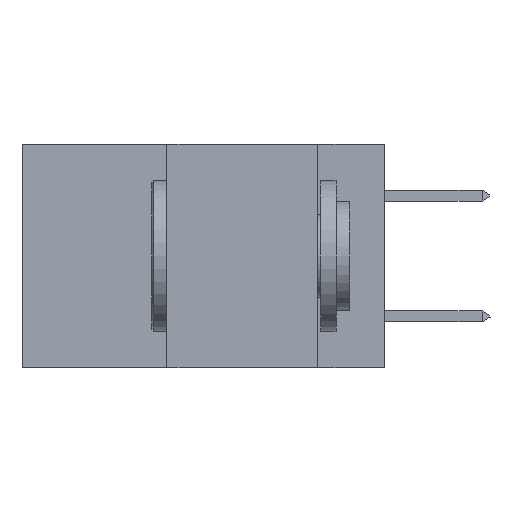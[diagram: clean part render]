
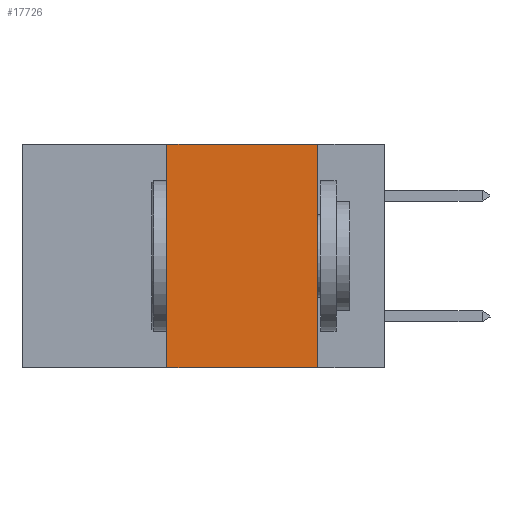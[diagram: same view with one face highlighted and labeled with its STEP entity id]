
A CAD part, left-side view. The second image highlights one B-rep face of the part: STEP entity #17726.
In plain terms, the highlighted planar face has unit normal (-1, 0, 0).
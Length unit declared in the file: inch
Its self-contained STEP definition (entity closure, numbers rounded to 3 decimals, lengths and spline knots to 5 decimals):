
#125 = LINE ( 'NONE', #22912, #5457 ) ;
#194 = ORIENTED_EDGE ( 'NONE', *, *, #4455, .F. ) ;
#486 = LINE ( 'NONE', #21158, #11023 ) ;
#777 = VERTEX_POINT ( 'NONE', #11724 ) ;
#1072 = EDGE_LOOP ( 'NONE', ( #14794, #11749, #194, #19528 ) ) ;
#1325 = EDGE_CURVE ( 'NONE', #26872, #3011, #125, .T. ) ;
#1342 = VECTOR ( 'NONE', #10791, 39.37008 ) ;
#3011 = VERTEX_POINT ( 'NONE', #22551 ) ;
#3086 = EDGE_CURVE ( 'NONE', #777, #14987, #8936, .T. ) ;
#4455 = EDGE_CURVE ( 'NONE', #777, #26872, #486, .T. ) ;
#4775 = CARTESIAN_POINT ( 'NONE',  ( 0., 0.11, -0.37 ) ) ;
#5297 = EDGE_CURVE ( 'NONE', #3011, #14987, #8090, .T. ) ;
#5457 = VECTOR ( 'NONE', #10984, 39.37008 ) ;
#8090 = LINE ( 'NONE', #26265, #26586 ) ;
#8412 = CARTESIAN_POINT ( 'NONE',  ( 0., 0.6, -0.37 ) ) ;
#8521 = CARTESIAN_POINT ( 'NONE',  ( 0., 0.36, 0. ) ) ;
#8615 = AXIS2_PLACEMENT_3D ( 'NONE', #26771, #11699, #13810 ) ;
#8936 = LINE ( 'NONE', #8412, #1342 ) ;
#10791 = DIRECTION ( 'NONE',  ( 0., -1., 0. ) ) ;
#10984 = DIRECTION ( 'NONE',  ( 0., -1., 0. ) ) ;
#11023 = VECTOR ( 'NONE', #14975, 39.37008 ) ;
#11699 = DIRECTION ( 'NONE',  ( 1., 0., 0. ) ) ;
#11724 = CARTESIAN_POINT ( 'NONE',  ( 0., 0.36, -0.37 ) ) ;
#11749 = ORIENTED_EDGE ( 'NONE', *, *, #1325, .F. ) ;
#12836 = FACE_OUTER_BOUND ( 'NONE', #1072, .T. ) ;
#13810 = DIRECTION ( 'NONE',  ( 0., 0., -1. ) ) ;
#13999 = PLANE ( 'NONE',  #8615 ) ;
#14794 = ORIENTED_EDGE ( 'NONE', *, *, #5297, .F. ) ;
#14975 = DIRECTION ( 'NONE',  ( 0., 0., 1. ) ) ;
#14987 = VERTEX_POINT ( 'NONE', #4775 ) ;
#17726 = ADVANCED_FACE ( 'NONE', ( #12836 ), #13999, .F. ) ;
#19528 = ORIENTED_EDGE ( 'NONE', *, *, #3086, .T. ) ;
#21158 = CARTESIAN_POINT ( 'NONE',  ( 0., 0.36, 0. ) ) ;
#22551 = CARTESIAN_POINT ( 'NONE',  ( 0., 0.11, 0. ) ) ;
#22912 = CARTESIAN_POINT ( 'NONE',  ( 0., 0.6, 0. ) ) ;
#23233 = DIRECTION ( 'NONE',  ( 0., 0., -1. ) ) ;
#26265 = CARTESIAN_POINT ( 'NONE',  ( 0., 0.11, 0. ) ) ;
#26586 = VECTOR ( 'NONE', #23233, 39.37008 ) ;
#26771 = CARTESIAN_POINT ( 'NONE',  ( 0., 0.6, 0. ) ) ;
#26872 = VERTEX_POINT ( 'NONE', #8521 ) ;
